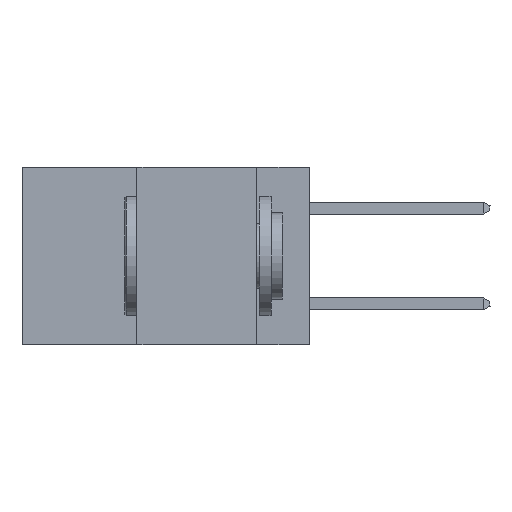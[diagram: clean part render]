
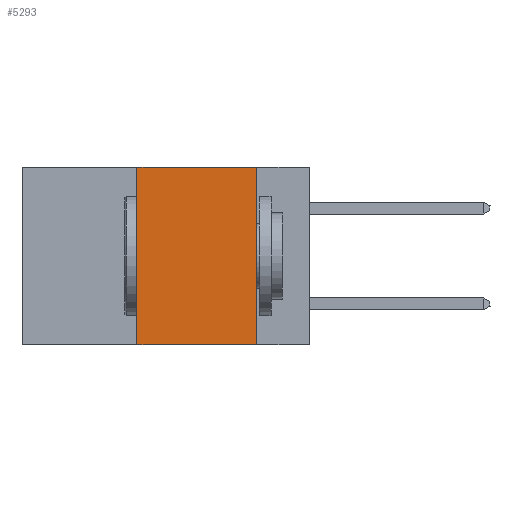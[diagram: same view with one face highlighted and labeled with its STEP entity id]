
A CAD part, left-side view. The second image highlights one B-rep face of the part: STEP entity #5293.
In plain terms, the highlighted planar face has unit normal (-1, 0, 0).
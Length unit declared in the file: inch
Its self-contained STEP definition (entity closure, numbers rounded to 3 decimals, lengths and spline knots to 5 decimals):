
#351 = CARTESIAN_POINT ( 'NONE',  ( 0., 0.36, 0. ) ) ;
#854 = LINE ( 'NONE', #2522, #23668 ) ;
#1332 = VERTEX_POINT ( 'NONE', #4952 ) ;
#2522 = CARTESIAN_POINT ( 'NONE',  ( 0., 0.11, 0. ) ) ;
#3650 = CARTESIAN_POINT ( 'NONE',  ( 0., 0.6, 0. ) ) ;
#4141 = VERTEX_POINT ( 'NONE', #21127 ) ;
#4668 = VECTOR ( 'NONE', #22252, 39.37008 ) ;
#4952 = CARTESIAN_POINT ( 'NONE',  ( 0., 0.36, -0.37 ) ) ;
#5197 = CARTESIAN_POINT ( 'NONE',  ( 0., 0.6, -0.37 ) ) ;
#5293 = ADVANCED_FACE ( 'NONE', ( #8958 ), #10170, .F. ) ;
#5861 = DIRECTION ( 'NONE',  ( 1., 0., 0. ) ) ;
#6974 = DIRECTION ( 'NONE',  ( 0., 0., -1. ) ) ;
#7145 = CARTESIAN_POINT ( 'NONE',  ( 0., 0.36, 0. ) ) ;
#7489 = VECTOR ( 'NONE', #13996, 39.37008 ) ;
#8442 = EDGE_CURVE ( 'NONE', #1332, #4141, #23904, .T. ) ;
#8844 = ORIENTED_EDGE ( 'NONE', *, *, #22589, .F. ) ;
#8958 = FACE_OUTER_BOUND ( 'NONE', #16249, .T. ) ;
#10170 = PLANE ( 'NONE',  #11561 ) ;
#11011 = EDGE_CURVE ( 'NONE', #1332, #19459, #25112, .T. ) ;
#11561 = AXIS2_PLACEMENT_3D ( 'NONE', #3650, #5861, #14755 ) ;
#13104 = CARTESIAN_POINT ( 'NONE',  ( 0., 0.6, 0. ) ) ;
#13614 = EDGE_CURVE ( 'NONE', #19459, #16006, #26431, .T. ) ;
#13996 = DIRECTION ( 'NONE',  ( 0., 0., 1. ) ) ;
#14244 = VECTOR ( 'NONE', #20639, 39.37008 ) ;
#14755 = DIRECTION ( 'NONE',  ( 0., 0., -1. ) ) ;
#14845 = CARTESIAN_POINT ( 'NONE',  ( 0., 0.11, 0. ) ) ;
#15882 = ORIENTED_EDGE ( 'NONE', *, *, #8442, .T. ) ;
#16006 = VERTEX_POINT ( 'NONE', #14845 ) ;
#16249 = EDGE_LOOP ( 'NONE', ( #8844, #19181, #18113, #15882 ) ) ;
#18113 = ORIENTED_EDGE ( 'NONE', *, *, #11011, .F. ) ;
#19181 = ORIENTED_EDGE ( 'NONE', *, *, #13614, .F. ) ;
#19459 = VERTEX_POINT ( 'NONE', #351 ) ;
#20639 = DIRECTION ( 'NONE',  ( 0., -1., 0. ) ) ;
#21127 = CARTESIAN_POINT ( 'NONE',  ( 0., 0.11, -0.37 ) ) ;
#22252 = DIRECTION ( 'NONE',  ( 0., -1., 0. ) ) ;
#22589 = EDGE_CURVE ( 'NONE', #16006, #4141, #854, .T. ) ;
#23668 = VECTOR ( 'NONE', #6974, 39.37008 ) ;
#23904 = LINE ( 'NONE', #5197, #14244 ) ;
#25112 = LINE ( 'NONE', #7145, #7489 ) ;
#26431 = LINE ( 'NONE', #13104, #4668 ) ;
